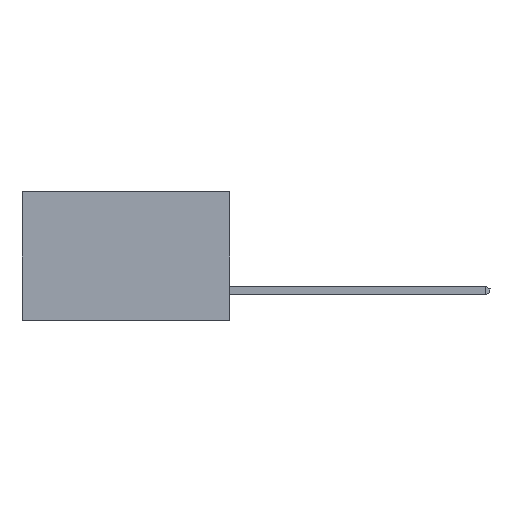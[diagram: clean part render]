
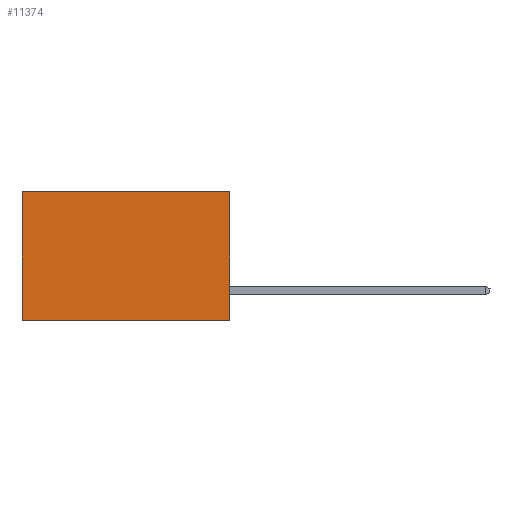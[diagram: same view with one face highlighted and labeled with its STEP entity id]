
A CAD part, left-side view. The second image highlights one B-rep face of the part: STEP entity #11374.
In plain terms, the highlighted planar face has unit normal (-1, 0, 0).
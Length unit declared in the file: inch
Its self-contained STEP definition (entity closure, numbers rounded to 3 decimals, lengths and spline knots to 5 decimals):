
#623 = CARTESIAN_POINT ( 'NONE',  ( 0.2615, 0., 0. ) ) ;
#1065 = DIRECTION ( 'NONE',  ( 1., 0., 0. ) ) ;
#2558 = EDGE_CURVE ( 'NONE', #2651, #9553, #7978, .T. ) ;
#2651 = VERTEX_POINT ( 'NONE', #15522 ) ;
#3178 = VECTOR ( 'NONE', #4168, 39.37008 ) ;
#3282 = CARTESIAN_POINT ( 'NONE',  ( 0.2615, 0.6, -0.37 ) ) ;
#3736 = CARTESIAN_POINT ( 'NONE',  ( 0.2615, 0.6, 0. ) ) ;
#3779 = VERTEX_POINT ( 'NONE', #5898 ) ;
#4168 = DIRECTION ( 'NONE',  ( 0., 0., -1. ) ) ;
#4822 = LINE ( 'NONE', #623, #5364 ) ;
#5083 = CARTESIAN_POINT ( 'NONE',  ( 0.2615, 0., -0.37 ) ) ;
#5364 = VECTOR ( 'NONE', #12353, 39.37008 ) ;
#5898 = CARTESIAN_POINT ( 'NONE',  ( 0.2615, 0.6, -0.37 ) ) ;
#6150 = CARTESIAN_POINT ( 'NONE',  ( 0.2615, 0., -0.37 ) ) ;
#6623 = VECTOR ( 'NONE', #15056, 39.37008 ) ;
#6692 = PLANE ( 'NONE',  #9571 ) ;
#7385 = EDGE_CURVE ( 'NONE', #10833, #3779, #15995, .T. ) ;
#7978 = LINE ( 'NONE', #5083, #17351 ) ;
#8432 = FACE_OUTER_BOUND ( 'NONE', #10858, .T. ) ;
#9553 = VERTEX_POINT ( 'NONE', #12931 ) ;
#9571 = AXIS2_PLACEMENT_3D ( 'NONE', #11326, #1065, #18508 ) ;
#10833 = VERTEX_POINT ( 'NONE', #3736 ) ;
#10858 = EDGE_LOOP ( 'NONE', ( #16082, #16314, #17728, #10931 ) ) ;
#10931 = ORIENTED_EDGE ( 'NONE', *, *, #15176, .T. ) ;
#11051 = DIRECTION ( 'NONE',  ( 0., 0., -1. ) ) ;
#11326 = CARTESIAN_POINT ( 'NONE',  ( 0.2615, 0., -0.37 ) ) ;
#11374 = ADVANCED_FACE ( 'NONE', ( #8432 ), #6692, .F. ) ;
#12353 = DIRECTION ( 'NONE',  ( 0., 1., 0. ) ) ;
#12931 = CARTESIAN_POINT ( 'NONE',  ( 0.2615, 0., -0.37 ) ) ;
#15056 = DIRECTION ( 'NONE',  ( 0., 1., 0. ) ) ;
#15176 = EDGE_CURVE ( 'NONE', #2651, #10833, #4822, .T. ) ;
#15522 = CARTESIAN_POINT ( 'NONE',  ( 0.2615, 0., 0. ) ) ;
#15995 = LINE ( 'NONE', #3282, #3178 ) ;
#16082 = ORIENTED_EDGE ( 'NONE', *, *, #7385, .T. ) ;
#16314 = ORIENTED_EDGE ( 'NONE', *, *, #18244, .F. ) ;
#17351 = VECTOR ( 'NONE', #11051, 39.37008 ) ;
#17728 = ORIENTED_EDGE ( 'NONE', *, *, #2558, .F. ) ;
#18165 = LINE ( 'NONE', #6150, #6623 ) ;
#18244 = EDGE_CURVE ( 'NONE', #9553, #3779, #18165, .T. ) ;
#18508 = DIRECTION ( 'NONE',  ( 0., 0., -1. ) ) ;
